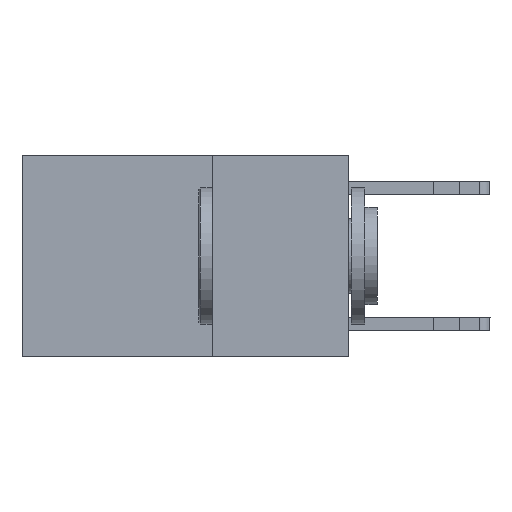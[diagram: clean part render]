
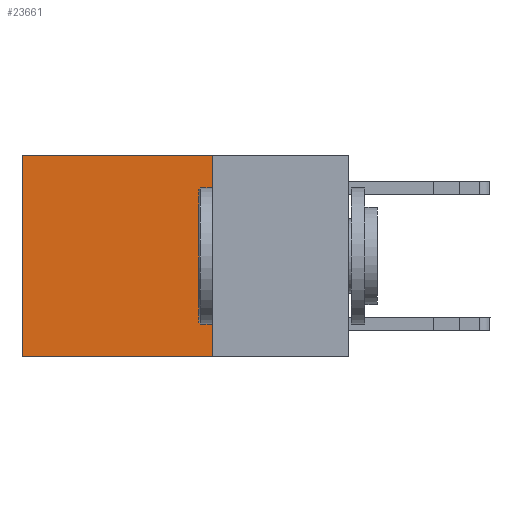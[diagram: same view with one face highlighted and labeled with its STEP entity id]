
A CAD part, left-side view. The second image highlights one B-rep face of the part: STEP entity #23661.
In plain terms, the highlighted planar face has unit normal (-1, 0, 0).
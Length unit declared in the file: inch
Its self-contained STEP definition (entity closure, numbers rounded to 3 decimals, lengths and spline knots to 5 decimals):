
#1184 = CARTESIAN_POINT ( 'NONE',  ( 0.2625, 0.25, 0. ) ) ;
#1572 = AXIS2_PLACEMENT_3D ( 'NONE', #25318, #3314, #18806 ) ;
#2760 = ORIENTED_EDGE ( 'NONE', *, *, #23685, .F. ) ;
#2775 = VERTEX_POINT ( 'NONE', #28192 ) ;
#2988 = EDGE_LOOP ( 'NONE', ( #16020, #13104, #2760, #9512 ) ) ;
#3314 = DIRECTION ( 'NONE',  ( 1., 0., 0. ) ) ;
#3401 = DIRECTION ( 'NONE',  ( 0., 0., -1. ) ) ;
#4280 = EDGE_CURVE ( 'NONE', #2775, #19729, #12378, .T. ) ;
#4705 = EDGE_CURVE ( 'NONE', #27074, #19729, #12349, .T. ) ;
#5456 = DIRECTION ( 'NONE',  ( 0., 1., 0. ) ) ;
#5562 = CARTESIAN_POINT ( 'NONE',  ( 0.2625, 0.25, 0. ) ) ;
#5784 = VECTOR ( 'NONE', #23438, 39.37008 ) ;
#7511 = VECTOR ( 'NONE', #3401, 39.37008 ) ;
#7655 = LINE ( 'NONE', #23041, #25945 ) ;
#9512 = ORIENTED_EDGE ( 'NONE', *, *, #16085, .T. ) ;
#10231 = CARTESIAN_POINT ( 'NONE',  ( 0.2625, 0.6, 0. ) ) ;
#10820 = CARTESIAN_POINT ( 'NONE',  ( 0.2625, 0.25, -0.37 ) ) ;
#12057 = DIRECTION ( 'NONE',  ( 0., 1., 0. ) ) ;
#12349 = LINE ( 'NONE', #20839, #17543 ) ;
#12378 = LINE ( 'NONE', #10231, #5784 ) ;
#12706 = LINE ( 'NONE', #1184, #7511 ) ;
#13104 = ORIENTED_EDGE ( 'NONE', *, *, #4705, .F. ) ;
#13913 = VERTEX_POINT ( 'NONE', #5562 ) ;
#16020 = ORIENTED_EDGE ( 'NONE', *, *, #4280, .T. ) ;
#16085 = EDGE_CURVE ( 'NONE', #13913, #2775, #7655, .T. ) ;
#16622 = PLANE ( 'NONE',  #1572 ) ;
#17543 = VECTOR ( 'NONE', #5456, 39.37008 ) ;
#18806 = DIRECTION ( 'NONE',  ( 0., 0., -1. ) ) ;
#19729 = VERTEX_POINT ( 'NONE', #25661 ) ;
#20839 = CARTESIAN_POINT ( 'NONE',  ( 0.2625, 0.25, -0.37 ) ) ;
#23041 = CARTESIAN_POINT ( 'NONE',  ( 0.2625, 0.25, 0. ) ) ;
#23438 = DIRECTION ( 'NONE',  ( 0., 0., -1. ) ) ;
#23661 = ADVANCED_FACE ( 'NONE', ( #24413 ), #16622, .F. ) ;
#23685 = EDGE_CURVE ( 'NONE', #13913, #27074, #12706, .T. ) ;
#24413 = FACE_OUTER_BOUND ( 'NONE', #2988, .T. ) ;
#25318 = CARTESIAN_POINT ( 'NONE',  ( 0.2625, 0.25, 0. ) ) ;
#25661 = CARTESIAN_POINT ( 'NONE',  ( 0.2625, 0.6, -0.37 ) ) ;
#25945 = VECTOR ( 'NONE', #12057, 39.37008 ) ;
#27074 = VERTEX_POINT ( 'NONE', #10820 ) ;
#28192 = CARTESIAN_POINT ( 'NONE',  ( 0.2625, 0.6, 0. ) ) ;
